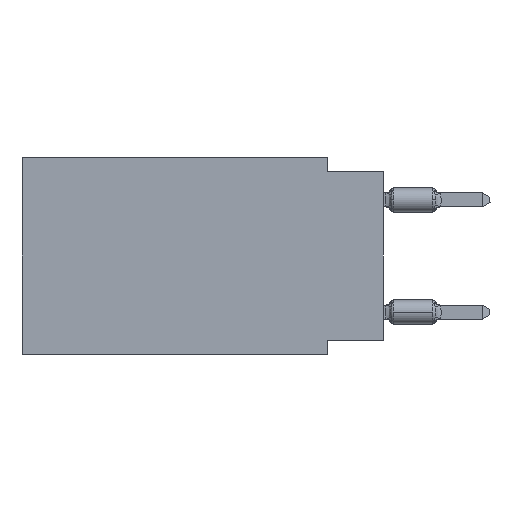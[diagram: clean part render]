
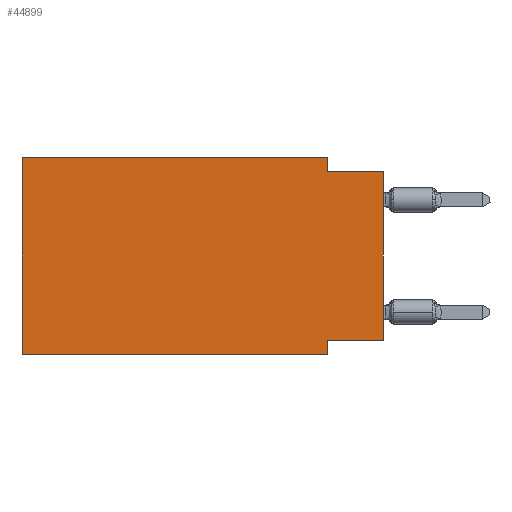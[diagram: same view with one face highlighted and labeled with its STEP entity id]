
A CAD part, left-side view. The second image highlights one B-rep face of the part: STEP entity #44899.
In plain terms, the highlighted planar face has unit normal (-1, 0, 0).
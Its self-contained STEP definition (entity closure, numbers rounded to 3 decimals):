
#321 = CARTESIAN_POINT ( 'NONE',  ( 0., 2.54, 0. ) ) ;
#1523 = EDGE_CURVE ( 'NONE', #39874, #18645, #25797, .T. ) ;
#1685 = ORIENTED_EDGE ( 'NONE', *, *, #4906, .F. ) ;
#2338 = EDGE_LOOP ( 'NONE', ( #30768, #31942, #20215, #20494, #1685, #53910, #15027, #20675 ) ) ;
#4906 = EDGE_CURVE ( 'NONE', #48999, #21804, #48442, .T. ) ;
#8358 = CARTESIAN_POINT ( 'NONE',  ( 0., 0., -8.255 ) ) ;
#8430 = DIRECTION ( 'NONE',  ( 0., 0., 1. ) ) ;
#8709 = CARTESIAN_POINT ( 'NONE',  ( 0., 16.383, 0. ) ) ;
#9544 = CARTESIAN_POINT ( 'NONE',  ( 0., 0., 0. ) ) ;
#10909 = VECTOR ( 'NONE', #21667, 1000. ) ;
#12095 = CARTESIAN_POINT ( 'NONE',  ( 0., 0., -8.255 ) ) ;
#13819 = CARTESIAN_POINT ( 'NONE',  ( 0., 16.383, 0. ) ) ;
#14163 = VECTOR ( 'NONE', #48606, 1000. ) ;
#14392 = DIRECTION ( 'NONE',  ( 0., -1., 0. ) ) ;
#15027 = ORIENTED_EDGE ( 'NONE', *, *, #1523, .F. ) ;
#15066 = VECTOR ( 'NONE', #14392, 1000. ) ;
#15757 = CARTESIAN_POINT ( 'NONE',  ( 0., 16.383, -8.89 ) ) ;
#16407 = CARTESIAN_POINT ( 'NONE',  ( 0., 2.54, -0.635 ) ) ;
#18645 = VERTEX_POINT ( 'NONE', #28360 ) ;
#19010 = DIRECTION ( 'NONE',  ( 0., -1., 0. ) ) ;
#19076 = EDGE_CURVE ( 'NONE', #48999, #18645, #23518, .T. ) ;
#20215 = ORIENTED_EDGE ( 'NONE', *, *, #55067, .F. ) ;
#20342 = AXIS2_PLACEMENT_3D ( 'NONE', #54202, #30675, #57748 ) ;
#20494 = ORIENTED_EDGE ( 'NONE', *, *, #27086, .F. ) ;
#20675 = ORIENTED_EDGE ( 'NONE', *, *, #43893, .F. ) ;
#21667 = DIRECTION ( 'NONE',  ( 0., 0., -1. ) ) ;
#21804 = VERTEX_POINT ( 'NONE', #13819 ) ;
#22138 = PLANE ( 'NONE',  #20342 ) ;
#23518 = LINE ( 'NONE', #41455, #15066 ) ;
#25797 = LINE ( 'NONE', #43735, #10909 ) ;
#25980 = CARTESIAN_POINT ( 'NONE',  ( 0., 2.54, -8.255 ) ) ;
#26267 = FACE_OUTER_BOUND ( 'NONE', #2338, .T. ) ;
#26481 = VERTEX_POINT ( 'NONE', #321 ) ;
#27086 = EDGE_CURVE ( 'NONE', #21804, #26481, #37863, .T. ) ;
#27780 = VECTOR ( 'NONE', #19010, 1000. ) ;
#28360 = CARTESIAN_POINT ( 'NONE',  ( 0., 2.54, -8.89 ) ) ;
#28869 = VERTEX_POINT ( 'NONE', #8358 ) ;
#30046 = DIRECTION ( 'NONE',  ( 0., 1., 0. ) ) ;
#30675 = DIRECTION ( 'NONE',  ( 1., 0., 0. ) ) ;
#30768 = ORIENTED_EDGE ( 'NONE', *, *, #44504, .T. ) ;
#31909 = LINE ( 'NONE', #9544, #32526 ) ;
#31942 = ORIENTED_EDGE ( 'NONE', *, *, #44146, .F. ) ;
#32526 = VECTOR ( 'NONE', #45437, 1000. ) ;
#34497 = VERTEX_POINT ( 'NONE', #36905 ) ;
#35343 = LINE ( 'NONE', #40047, #14163 ) ;
#35931 = VECTOR ( 'NONE', #42578, 1000. ) ;
#36905 = CARTESIAN_POINT ( 'NONE',  ( 0., 0., -0.635 ) ) ;
#37139 = VECTOR ( 'NONE', #30046, 1000. ) ;
#37863 = LINE ( 'NONE', #42297, #35931 ) ;
#39241 = VECTOR ( 'NONE', #8430, 1000. ) ;
#39874 = VERTEX_POINT ( 'NONE', #25980 ) ;
#40047 = CARTESIAN_POINT ( 'NONE',  ( 0., 2.54, 0. ) ) ;
#41455 = CARTESIAN_POINT ( 'NONE',  ( 0., 16.383, -8.89 ) ) ;
#42297 = CARTESIAN_POINT ( 'NONE',  ( 0., 16.383, 0. ) ) ;
#42578 = DIRECTION ( 'NONE',  ( 0., -1., 0. ) ) ;
#43735 = CARTESIAN_POINT ( 'NONE',  ( 0., 2.54, -8.89 ) ) ;
#43893 = EDGE_CURVE ( 'NONE', #28869, #39874, #52408, .T. ) ;
#44146 = EDGE_CURVE ( 'NONE', #56968, #34497, #54915, .T. ) ;
#44504 = EDGE_CURVE ( 'NONE', #28869, #34497, #31909, .T. ) ;
#44899 = ADVANCED_FACE ( 'NONE', ( #26267 ), #22138, .F. ) ;
#45437 = DIRECTION ( 'NONE',  ( 0., 0., 1. ) ) ;
#48442 = LINE ( 'NONE', #8709, #39241 ) ;
#48606 = DIRECTION ( 'NONE',  ( 0., 0., -1. ) ) ;
#48999 = VERTEX_POINT ( 'NONE', #15757 ) ;
#52408 = LINE ( 'NONE', #12095, #37139 ) ;
#53910 = ORIENTED_EDGE ( 'NONE', *, *, #19076, .T. ) ;
#54202 = CARTESIAN_POINT ( 'NONE',  ( 0., 16.383, 0. ) ) ;
#54915 = LINE ( 'NONE', #55781, #27780 ) ;
#55067 = EDGE_CURVE ( 'NONE', #26481, #56968, #35343, .T. ) ;
#55781 = CARTESIAN_POINT ( 'NONE',  ( 0., 0., -0.635 ) ) ;
#56968 = VERTEX_POINT ( 'NONE', #16407 ) ;
#57748 = DIRECTION ( 'NONE',  ( 0., 0., -1. ) ) ;
